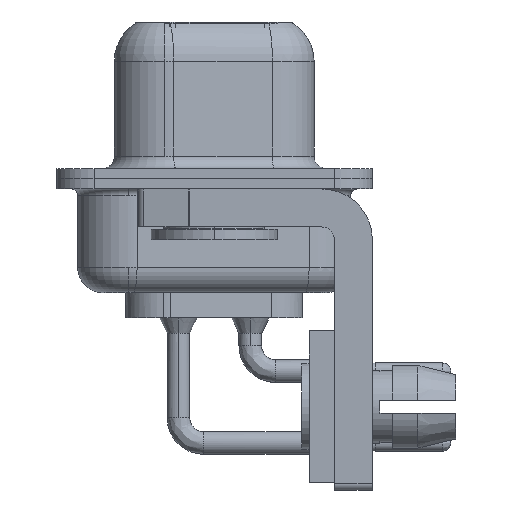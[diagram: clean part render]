
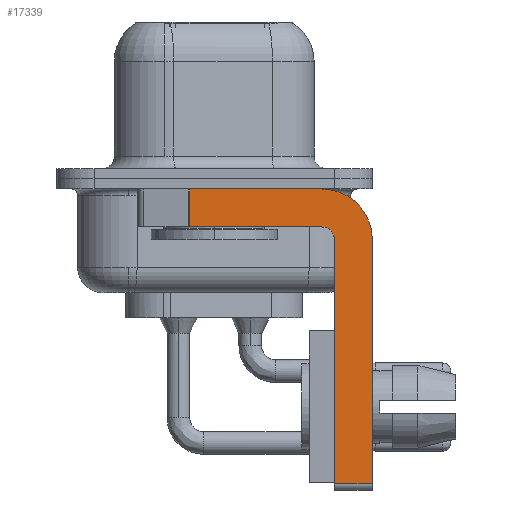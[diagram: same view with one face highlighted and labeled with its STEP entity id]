
A CAD part, left-side view. The second image highlights one B-rep face of the part: STEP entity #17339.
In plain terms, the highlighted planar face has unit normal (-1, 0, 0).
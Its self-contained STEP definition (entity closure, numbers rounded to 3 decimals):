
#149 = CARTESIAN_POINT ( 'NONE',  ( -2.9, -6.25, -12.05 ) ) ;
#653 = DIRECTION ( 'NONE',  ( 0., 1., 0. ) ) ;
#890 = VERTEX_POINT ( 'NONE', #6390 ) ;
#1269 = CARTESIAN_POINT ( 'NONE',  ( -2.9, -4.25, -2.4 ) ) ;
#1417 = EDGE_CURVE ( 'NONE', #4147, #8763, #18826, .T. ) ;
#1498 = CARTESIAN_POINT ( 'NONE',  ( -2.9, -4.25, -0.4 ) ) ;
#2392 = DIRECTION ( 'NONE',  ( -1., 0., 0. ) ) ;
#3023 = CARTESIAN_POINT ( 'NONE',  ( -2.9, 0.978, -0.4 ) ) ;
#3334 = DIRECTION ( 'NONE',  ( 1., 0., 0. ) ) ;
#3455 = VERTEX_POINT ( 'NONE', #21836 ) ;
#4147 = VERTEX_POINT ( 'NONE', #3023 ) ;
#4406 = ORIENTED_EDGE ( 'NONE', *, *, #10586, .T. ) ;
#4522 = DIRECTION ( 'NONE',  ( 0., 0., -1. ) ) ;
#6390 = CARTESIAN_POINT ( 'NONE',  ( -2.9, -4.25, -1.9 ) ) ;
#6392 = VECTOR ( 'NONE', #23677, 1000. ) ;
#6794 = CIRCLE ( 'NONE', #15451, 2. ) ;
#7313 = CARTESIAN_POINT ( 'NONE',  ( -2.9, -4.75, -2.4 ) ) ;
#8336 = EDGE_LOOP ( 'NONE', ( #22797, #4406, #10164, #20635, #8591, #14365, #16944, #19839 ) ) ;
#8435 = AXIS2_PLACEMENT_3D ( 'NONE', #14662, #2392, #16691 ) ;
#8473 = DIRECTION ( 'NONE',  ( 0., 0., -1. ) ) ;
#8519 = CARTESIAN_POINT ( 'NONE',  ( -2.9, -6.25, -2.4 ) ) ;
#8591 = ORIENTED_EDGE ( 'NONE', *, *, #13866, .F. ) ;
#8763 = VERTEX_POINT ( 'NONE', #1498 ) ;
#9436 = CARTESIAN_POINT ( 'NONE',  ( -2.9, -4.75, -12.3 ) ) ;
#9521 = DIRECTION ( 'NONE',  ( 1., 0., 0. ) ) ;
#9627 = VERTEX_POINT ( 'NONE', #8519 ) ;
#10164 = ORIENTED_EDGE ( 'NONE', *, *, #21909, .F. ) ;
#10370 = CARTESIAN_POINT ( 'NONE',  ( -2.9, 3., -0.4 ) ) ;
#10586 = EDGE_CURVE ( 'NONE', #4147, #3455, #14507, .T. ) ;
#11478 = DIRECTION ( 'NONE',  ( 0., 0., 1. ) ) ;
#12075 = EDGE_CURVE ( 'NONE', #8763, #9627, #6794, .T. ) ;
#13475 = VECTOR ( 'NONE', #18029, 1000. ) ;
#13639 = LINE ( 'NONE', #23235, #23884 ) ;
#13866 = EDGE_CURVE ( 'NONE', #17119, #15505, #15349, .T. ) ;
#14365 = ORIENTED_EDGE ( 'NONE', *, *, #14848, .T. ) ;
#14507 = LINE ( 'NONE', #20629, #25431 ) ;
#14662 = CARTESIAN_POINT ( 'NONE',  ( -2.9, -4.25, -2.4 ) ) ;
#14848 = EDGE_CURVE ( 'NONE', #17119, #16115, #17193, .T. ) ;
#14996 = CARTESIAN_POINT ( 'NONE',  ( -2.9, -4.75, -12.05 ) ) ;
#15066 = CIRCLE ( 'NONE', #8435, 0.5 ) ;
#15349 = LINE ( 'NONE', #9436, #25643 ) ;
#15451 = AXIS2_PLACEMENT_3D ( 'NONE', #21707, #9521, #23798 ) ;
#15505 = VERTEX_POINT ( 'NONE', #7313 ) ;
#16115 = VERTEX_POINT ( 'NONE', #149 ) ;
#16691 = DIRECTION ( 'NONE',  ( 0., 0., 1. ) ) ;
#16944 = ORIENTED_EDGE ( 'NONE', *, *, #22468, .F. ) ;
#17119 = VERTEX_POINT ( 'NONE', #14996 ) ;
#17193 = LINE ( 'NONE', #21583, #6392 ) ;
#17236 = AXIS2_PLACEMENT_3D ( 'NONE', #1269, #3334, #17638 ) ;
#17318 = FACE_OUTER_BOUND ( 'NONE', #8336, .T. ) ;
#17339 = ADVANCED_FACE ( 'NONE', ( #17318 ), #17543, .F. ) ;
#17543 = PLANE ( 'NONE',  #17236 ) ;
#17638 = DIRECTION ( 'NONE',  ( 0., 0., -1. ) ) ;
#18029 = DIRECTION ( 'NONE',  ( 0., -1., 0. ) ) ;
#18295 = EDGE_CURVE ( 'NONE', #15505, #890, #15066, .T. ) ;
#18773 = CARTESIAN_POINT ( 'NONE',  ( -2.9, -6.25, -2.4 ) ) ;
#18826 = LINE ( 'NONE', #10370, #13475 ) ;
#19839 = ORIENTED_EDGE ( 'NONE', *, *, #12075, .F. ) ;
#20629 = CARTESIAN_POINT ( 'NONE',  ( -2.9, 0.978, -1.9 ) ) ;
#20635 = ORIENTED_EDGE ( 'NONE', *, *, #18295, .F. ) ;
#21583 = CARTESIAN_POINT ( 'NONE',  ( -2.9, -4.25, -12.05 ) ) ;
#21707 = CARTESIAN_POINT ( 'NONE',  ( -2.9, -4.25, -2.4 ) ) ;
#21836 = CARTESIAN_POINT ( 'NONE',  ( -2.9, 0.978, -1.9 ) ) ;
#21909 = EDGE_CURVE ( 'NONE', #890, #3455, #13639, .T. ) ;
#22468 = EDGE_CURVE ( 'NONE', #9627, #16115, #24499, .T. ) ;
#22797 = ORIENTED_EDGE ( 'NONE', *, *, #1417, .F. ) ;
#23196 = VECTOR ( 'NONE', #4522, 1000. ) ;
#23235 = CARTESIAN_POINT ( 'NONE',  ( -2.9, -4.25, -1.9 ) ) ;
#23677 = DIRECTION ( 'NONE',  ( 0., -1., 0. ) ) ;
#23798 = DIRECTION ( 'NONE',  ( 0., 0., -1. ) ) ;
#23884 = VECTOR ( 'NONE', #653, 1000. ) ;
#24499 = LINE ( 'NONE', #18773, #23196 ) ;
#25431 = VECTOR ( 'NONE', #8473, 1000. ) ;
#25643 = VECTOR ( 'NONE', #11478, 1000. ) ;
